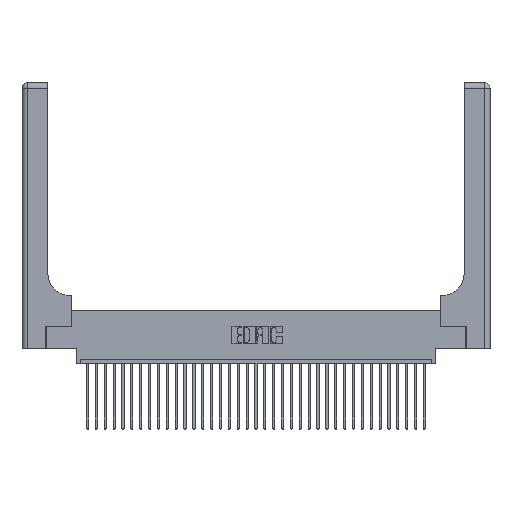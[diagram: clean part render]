
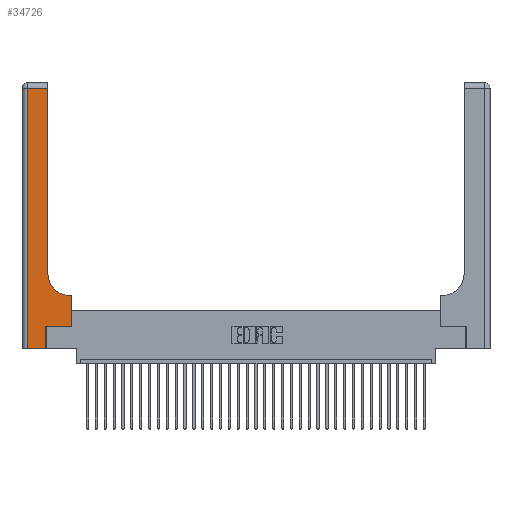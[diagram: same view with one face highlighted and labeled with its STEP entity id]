
A CAD part, top view. The second image highlights one B-rep face of the part: STEP entity #34726.
In plain terms, the highlighted planar face has unit normal (0, 0, 1).
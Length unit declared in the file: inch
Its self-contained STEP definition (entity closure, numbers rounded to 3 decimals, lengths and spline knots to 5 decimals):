
#156 = ORIENTED_EDGE ( 'NONE', *, *, #21807, .T. ) ;
#566 = CARTESIAN_POINT ( 'NONE',  ( 0.06, 2.94, 0.37 ) ) ;
#1589 = CARTESIAN_POINT ( 'NONE',  ( 0.269, 0.25, 0.37 ) ) ;
#1594 = EDGE_CURVE ( 'NONE', #18940, #29490, #32516, .T. ) ;
#3042 = LINE ( 'NONE', #30194, #10711 ) ;
#3140 = CARTESIAN_POINT ( 'NONE',  ( 0.5585, 0.25, 0.37 ) ) ;
#3338 = EDGE_CURVE ( 'NONE', #9725, #8008, #6888, .T. ) ;
#3668 = ORIENTED_EDGE ( 'NONE', *, *, #35115, .T. ) ;
#3797 = ORIENTED_EDGE ( 'NONE', *, *, #5664, .T. ) ;
#4008 = DIRECTION ( 'NONE',  ( 0., 1., 0. ) ) ;
#4285 = VECTOR ( 'NONE', #16802, 39.37008 ) ;
#4703 = VECTOR ( 'NONE', #21973, 39.37008 ) ;
#5664 = EDGE_CURVE ( 'NONE', #8008, #23244, #14350, .T. ) ;
#6219 = DIRECTION ( 'NONE',  ( 1., 0., 0. ) ) ;
#6666 = CARTESIAN_POINT ( 'NONE',  ( 0.2915, 0.85, 0.37 ) ) ;
#6872 = CARTESIAN_POINT ( 'NONE',  ( 0.5585, 0.6, 0.37 ) ) ;
#6888 = LINE ( 'NONE', #7683, #18285 ) ;
#7642 = CARTESIAN_POINT ( 'NONE',  ( 0.06, 3., 0.37 ) ) ;
#7683 = CARTESIAN_POINT ( 'NONE',  ( 0.269, 0., 0.37 ) ) ;
#7789 = VERTEX_POINT ( 'NONE', #24859 ) ;
#8008 = VERTEX_POINT ( 'NONE', #1589 ) ;
#8800 = VECTOR ( 'NONE', #25381, 39.37008 ) ;
#8916 = ORIENTED_EDGE ( 'NONE', *, *, #31083, .T. ) ;
#9725 = VERTEX_POINT ( 'NONE', #10728 ) ;
#9912 = VECTOR ( 'NONE', #24882, 39.37008 ) ;
#10018 = VECTOR ( 'NONE', #34198, 39.37008 ) ;
#10711 = VECTOR ( 'NONE', #25205, 39.37008 ) ;
#10728 = CARTESIAN_POINT ( 'NONE',  ( 0.269, 0., 0.37 ) ) ;
#11795 = EDGE_CURVE ( 'NONE', #30208, #25401, #23653, .T. ) ;
#12316 = CARTESIAN_POINT ( 'NONE',  ( 0., 3., 0.37 ) ) ;
#12977 = CARTESIAN_POINT ( 'NONE',  ( 0.5585, 0.25, 0.37 ) ) ;
#14306 = PLANE ( 'NONE',  #20742 ) ;
#14350 = LINE ( 'NONE', #22653, #8800 ) ;
#14591 = AXIS2_PLACEMENT_3D ( 'NONE', #27831, #16697, #6219 ) ;
#14806 = LINE ( 'NONE', #33401, #4703 ) ;
#15356 = DIRECTION ( 'NONE',  ( 0., 0., -1. ) ) ;
#16374 = ORIENTED_EDGE ( 'NONE', *, *, #1594, .T. ) ;
#16697 = DIRECTION ( 'NONE',  ( 0., 0., -1. ) ) ;
#16802 = DIRECTION ( 'NONE',  ( -1., 0., 0. ) ) ;
#17701 = DIRECTION ( 'NONE',  ( -1., 0., 0. ) ) ;
#18285 = VECTOR ( 'NONE', #23751, 39.37008 ) ;
#18940 = VERTEX_POINT ( 'NONE', #566 ) ;
#19638 = CARTESIAN_POINT ( 'NONE',  ( 0., 2.94, 0.37 ) ) ;
#20042 = FACE_OUTER_BOUND ( 'NONE', #23073, .T. ) ;
#20246 = LINE ( 'NONE', #31475, #32997 ) ;
#20742 = AXIS2_PLACEMENT_3D ( 'NONE', #12316, #15356, #17701 ) ;
#21807 = EDGE_CURVE ( 'NONE', #23869, #30208, #14806, .T. ) ;
#21973 = DIRECTION ( 'NONE',  ( -1., 0., 0. ) ) ;
#22572 = EDGE_CURVE ( 'NONE', #25401, #7789, #20246, .T. ) ;
#22619 = ORIENTED_EDGE ( 'NONE', *, *, #11795, .T. ) ;
#22653 = CARTESIAN_POINT ( 'NONE',  ( 0.269, 0.25, 0.37 ) ) ;
#23073 = EDGE_LOOP ( 'NONE', ( #31326, #29721, #16374, #8916, #33968, #3797, #3668, #156, #22619 ) ) ;
#23244 = VERTEX_POINT ( 'NONE', #12977 ) ;
#23653 = CIRCLE ( 'NONE', #14591, 0.25 ) ;
#23751 = DIRECTION ( 'NONE',  ( 0., 1., 0. ) ) ;
#23869 = VERTEX_POINT ( 'NONE', #6872 ) ;
#24859 = CARTESIAN_POINT ( 'NONE',  ( 0.2915, 2.94, 0.37 ) ) ;
#24882 = DIRECTION ( 'NONE',  ( 0., 1., 0. ) ) ;
#25119 = LINE ( 'NONE', #3140, #9912 ) ;
#25205 = DIRECTION ( 'NONE',  ( 1., 0., 0. ) ) ;
#25381 = DIRECTION ( 'NONE',  ( 1., 0., 0. ) ) ;
#25401 = VERTEX_POINT ( 'NONE', #6666 ) ;
#27831 = CARTESIAN_POINT ( 'NONE',  ( 0.5415, 0.85, 0.37 ) ) ;
#29490 = VERTEX_POINT ( 'NONE', #31686 ) ;
#29721 = ORIENTED_EDGE ( 'NONE', *, *, #32406, .T. ) ;
#29817 = CARTESIAN_POINT ( 'NONE',  ( 0.5415, 0.6, 0.37 ) ) ;
#30194 = CARTESIAN_POINT ( 'NONE',  ( 0., 0., 0.37 ) ) ;
#30208 = VERTEX_POINT ( 'NONE', #29817 ) ;
#31083 = EDGE_CURVE ( 'NONE', #29490, #9725, #3042, .T. ) ;
#31326 = ORIENTED_EDGE ( 'NONE', *, *, #22572, .T. ) ;
#31475 = CARTESIAN_POINT ( 'NONE',  ( 0.2915, 3., 0.37 ) ) ;
#31686 = CARTESIAN_POINT ( 'NONE',  ( 0.06, 0., 0.37 ) ) ;
#32406 = EDGE_CURVE ( 'NONE', #7789, #18940, #32651, .T. ) ;
#32516 = LINE ( 'NONE', #7642, #10018 ) ;
#32651 = LINE ( 'NONE', #19638, #4285 ) ;
#32997 = VECTOR ( 'NONE', #4008, 39.37008 ) ;
#33401 = CARTESIAN_POINT ( 'NONE',  ( 0.2915, 0.6, 0.37 ) ) ;
#33968 = ORIENTED_EDGE ( 'NONE', *, *, #3338, .T. ) ;
#34198 = DIRECTION ( 'NONE',  ( 0., -1., 0. ) ) ;
#34726 = ADVANCED_FACE ( 'NONE', ( #20042 ), #14306, .F. ) ;
#35115 = EDGE_CURVE ( 'NONE', #23244, #23869, #25119, .T. ) ;
